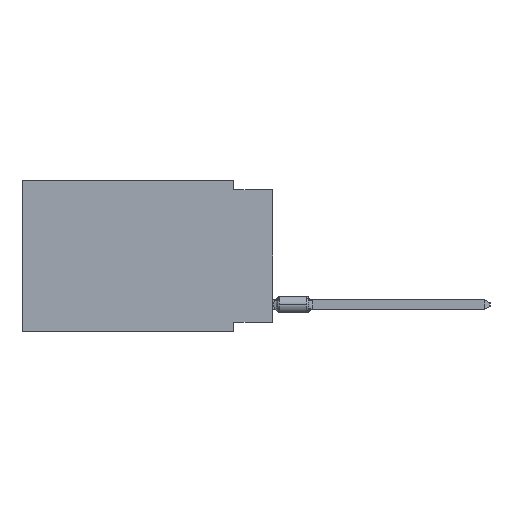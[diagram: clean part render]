
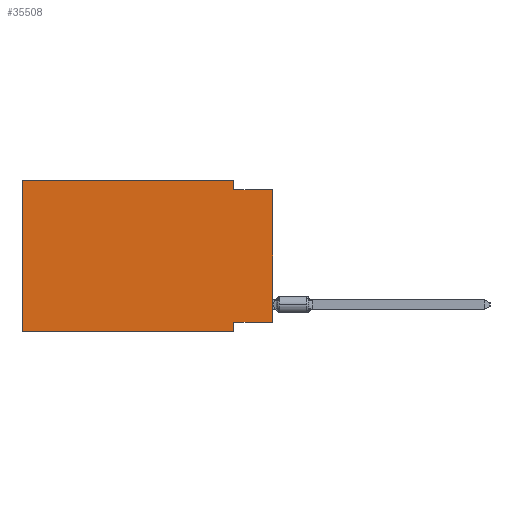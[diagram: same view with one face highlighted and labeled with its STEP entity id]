
A CAD part, left-side view. The second image highlights one B-rep face of the part: STEP entity #35508.
In plain terms, the highlighted planar face has unit normal (-1, 0, 0).
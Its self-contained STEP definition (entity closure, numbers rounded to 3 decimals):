
#1416 = EDGE_CURVE ( 'NONE', #21266, #20063, #66831, .T. ) ;
#2049 = VERTEX_POINT ( 'NONE', #28011 ) ;
#3020 = DIRECTION ( 'NONE',  ( 0., 0., -1. ) ) ;
#3280 = CARTESIAN_POINT ( 'NONE',  ( 0., 0., -0.635 ) ) ;
#3927 = ORIENTED_EDGE ( 'NONE', *, *, #28903, .T. ) ;
#5368 = VECTOR ( 'NONE', #24894, 1000. ) ;
#6559 = ORIENTED_EDGE ( 'NONE', *, *, #57723, .F. ) ;
#6904 = LINE ( 'NONE', #54010, #5368 ) ;
#6943 = ORIENTED_EDGE ( 'NONE', *, *, #53616, .F. ) ;
#7654 = VECTOR ( 'NONE', #42773, 1000. ) ;
#7740 = LINE ( 'NONE', #11998, #52697 ) ;
#11982 = DIRECTION ( 'NONE',  ( 1., 0., 0. ) ) ;
#11998 = CARTESIAN_POINT ( 'NONE',  ( 0., 2.54, 0. ) ) ;
#12838 = VECTOR ( 'NONE', #54768, 1000. ) ;
#12903 = CARTESIAN_POINT ( 'NONE',  ( 0., 16.383, -9.906 ) ) ;
#13420 = LINE ( 'NONE', #71673, #12838 ) ;
#13451 = EDGE_CURVE ( 'NONE', #26235, #36074, #29860, .T. ) ;
#16554 = EDGE_CURVE ( 'NONE', #61043, #26063, #7740, .T. ) ;
#17091 = ORIENTED_EDGE ( 'NONE', *, *, #16554, .F. ) ;
#17580 = EDGE_CURVE ( 'NONE', #20063, #61043, #31092, .T. ) ;
#17723 = PLANE ( 'NONE',  #41145 ) ;
#20063 = VERTEX_POINT ( 'NONE', #47678 ) ;
#21266 = VERTEX_POINT ( 'NONE', #25824 ) ;
#24158 = VERTEX_POINT ( 'NONE', #3280 ) ;
#24894 = DIRECTION ( 'NONE',  ( 0., -1., 0. ) ) ;
#24936 = DIRECTION ( 'NONE',  ( 0., -1., 0. ) ) ;
#25124 = LINE ( 'NONE', #12903, #7654 ) ;
#25824 = CARTESIAN_POINT ( 'NONE',  ( 0., 16.383, -9.906 ) ) ;
#26063 = VERTEX_POINT ( 'NONE', #57718 ) ;
#26235 = VERTEX_POINT ( 'NONE', #67639 ) ;
#26376 = CARTESIAN_POINT ( 'NONE',  ( 0., 2.54, -9.906 ) ) ;
#28011 = CARTESIAN_POINT ( 'NONE',  ( 0., 2.54, -9.906 ) ) ;
#28903 = EDGE_CURVE ( 'NONE', #21266, #2049, #25124, .T. ) ;
#29521 = EDGE_CURVE ( 'NONE', #26235, #24158, #13420, .T. ) ;
#29860 = LINE ( 'NONE', #53202, #54828 ) ;
#31092 = LINE ( 'NONE', #37612, #69971 ) ;
#31982 = ORIENTED_EDGE ( 'NONE', *, *, #13451, .F. ) ;
#35356 = DIRECTION ( 'NONE',  ( 0., 0., -1. ) ) ;
#35508 = ADVANCED_FACE ( 'NONE', ( #52576 ), #17723, .F. ) ;
#35531 = ORIENTED_EDGE ( 'NONE', *, *, #29521, .T. ) ;
#36074 = VERTEX_POINT ( 'NONE', #37918 ) ;
#37167 = VECTOR ( 'NONE', #67212, 1000. ) ;
#37612 = CARTESIAN_POINT ( 'NONE',  ( 0., 16.383, 0. ) ) ;
#37918 = CARTESIAN_POINT ( 'NONE',  ( 0., 2.54, -9.271 ) ) ;
#41145 = AXIS2_PLACEMENT_3D ( 'NONE', #64466, #11982, #35356 ) ;
#42773 = DIRECTION ( 'NONE',  ( 0., -1., 0. ) ) ;
#47678 = CARTESIAN_POINT ( 'NONE',  ( 0., 16.383, 0. ) ) ;
#48126 = EDGE_LOOP ( 'NONE', ( #35531, #6943, #17091, #66853, #58530, #3927, #6559, #31982 ) ) ;
#49817 = VECTOR ( 'NONE', #3020, 1000. ) ;
#52104 = DIRECTION ( 'NONE',  ( 0., 1., 0. ) ) ;
#52576 = FACE_OUTER_BOUND ( 'NONE', #48126, .T. ) ;
#52697 = VECTOR ( 'NONE', #59842, 1000. ) ;
#53202 = CARTESIAN_POINT ( 'NONE',  ( 0., 0., -9.271 ) ) ;
#53616 = EDGE_CURVE ( 'NONE', #26063, #24158, #6904, .T. ) ;
#54010 = CARTESIAN_POINT ( 'NONE',  ( 0., 0., -0.635 ) ) ;
#54768 = DIRECTION ( 'NONE',  ( 0., 0., 1. ) ) ;
#54828 = VECTOR ( 'NONE', #52104, 1000. ) ;
#56425 = CARTESIAN_POINT ( 'NONE',  ( 0., 2.54, 0. ) ) ;
#57718 = CARTESIAN_POINT ( 'NONE',  ( 0., 2.54, -0.635 ) ) ;
#57723 = EDGE_CURVE ( 'NONE', #36074, #2049, #62019, .T. ) ;
#58530 = ORIENTED_EDGE ( 'NONE', *, *, #1416, .F. ) ;
#59842 = DIRECTION ( 'NONE',  ( 0., 0., -1. ) ) ;
#61043 = VERTEX_POINT ( 'NONE', #56425 ) ;
#62019 = LINE ( 'NONE', #26376, #49817 ) ;
#64466 = CARTESIAN_POINT ( 'NONE',  ( 0., 16.383, 0. ) ) ;
#66831 = LINE ( 'NONE', #72971, #37167 ) ;
#66853 = ORIENTED_EDGE ( 'NONE', *, *, #17580, .F. ) ;
#67212 = DIRECTION ( 'NONE',  ( 0., 0., 1. ) ) ;
#67639 = CARTESIAN_POINT ( 'NONE',  ( 0., 0., -9.271 ) ) ;
#69971 = VECTOR ( 'NONE', #24936, 1000. ) ;
#71673 = CARTESIAN_POINT ( 'NONE',  ( 0., 0., 0. ) ) ;
#72971 = CARTESIAN_POINT ( 'NONE',  ( 0., 16.383, 0. ) ) ;
